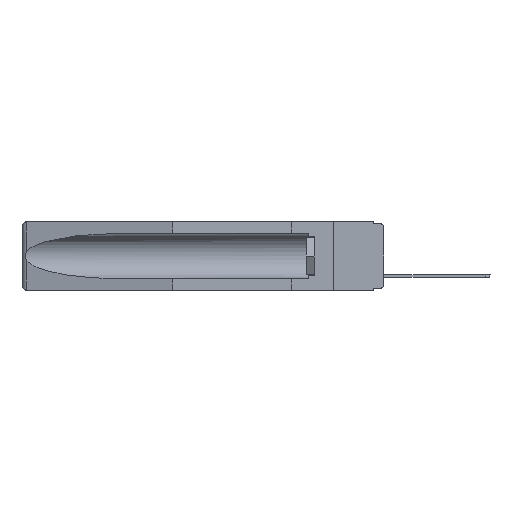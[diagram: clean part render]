
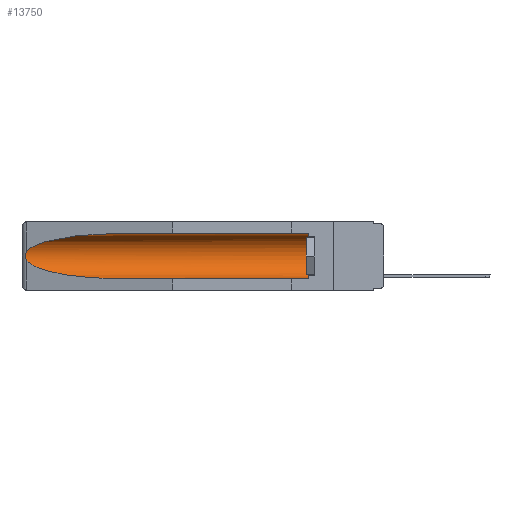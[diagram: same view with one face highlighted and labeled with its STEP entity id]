
A CAD part, left-side view. The second image highlights one B-rep face of the part: STEP entity #13750.
In plain terms, the highlighted cylindrical face has radius 2.857 mm (diameter 5.715 mm), a partial arc.
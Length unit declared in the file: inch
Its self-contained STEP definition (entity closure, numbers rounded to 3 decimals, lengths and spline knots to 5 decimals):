
#1207 = DIRECTION ( 'NONE',  ( 0., 0., 1. ) ) ;
#1569 = ORIENTED_EDGE ( 'NONE', *, *, #2004, .T. ) ;
#1913 = VERTEX_POINT ( 'NONE', #12343 ) ;
#1918 = CARTESIAN_POINT ( 'NONE',  ( 0.155, 1.07973, -0.059 ) ) ;
#1932 = EDGE_CURVE ( 'NONE', #7991, #20715, #3183, .T. ) ;
#2004 = EDGE_CURVE ( 'NONE', #13386, #7965, #2356, .T. ) ;
#2179 = CARTESIAN_POINT ( 'NONE',  ( 0.2673, 1.53269, -0.17917 ) ) ;
#2356 =( BOUNDED_CURVE ( )  B_SPLINE_CURVE ( 3, ( #19872, #16302, #10547, #3403 ),
 .UNSPECIFIED., .F., .F. ) 
 B_SPLINE_CURVE_WITH_KNOTS ( ( 4, 4 ),
 ( 0.1948, 1.5708 ),
 .UNSPECIFIED. ) 
 CURVE ( )  GEOMETRIC_REPRESENTATION_ITEM ( )  RATIONAL_B_SPLINE_CURVE ( ( 1., 0.848, 0.848, 1. ) ) 
 REPRESENTATION_ITEM ( '' )  );
#2680 = VECTOR ( 'NONE', #16336, 39.37008 ) ;
#2897 = DIRECTION ( 'NONE',  ( 0., 0., 1. ) ) ;
#3183 = LINE ( 'NONE', #8618, #13133 ) ;
#3218 = LINE ( 'NONE', #8899, #2680 ) ;
#3403 = CARTESIAN_POINT ( 'NONE',  ( 0.155, 1.07973, -0.284 ) ) ;
#3861 = CARTESIAN_POINT ( 'NONE',  ( 0.2673, 1.5327, -0.16383 ) ) ;
#4506 = DIRECTION ( 'NONE',  ( 0., 1., 0. ) ) ;
#5332 = AXIS2_PLACEMENT_3D ( 'NONE', #14336, #21502, #1207 ) ;
#5434 = CARTESIAN_POINT ( 'NONE',  ( 0.2675, 1.53308, -0.16763 ) ) ;
#5919 = CARTESIAN_POINT ( 'NONE',  ( 0.26597, 1.5296, -0.19026 ) ) ;
#7965 = VERTEX_POINT ( 'NONE', #21753 ) ;
#7991 = VERTEX_POINT ( 'NONE', #19825 ) ;
#8219 = B_SPLINE_CURVE_WITH_KNOTS ( 'NONE', 3,
 ( #22138, #22256, #20326, #3861, #5434, #18418, #2179, #18542, #5919, #16748 ),
 .UNSPECIFIED., .F., .F.,
 ( 4, 2, 2, 2, 4 ),
 ( 0., 0.00029, 0.00058, 0.00087, 0.00117 ),
 .UNSPECIFIED. ) ;
#8432 = CARTESIAN_POINT ( 'NONE',  ( 0.155, 0.126, -0.1715 ) ) ;
#8453 = CIRCLE ( 'NONE', #15736, 0.1125 ) ;
#8618 = CARTESIAN_POINT ( 'NONE',  ( 0.155, -0.30754, -0.059 ) ) ;
#8899 = CARTESIAN_POINT ( 'NONE',  ( 0.155, -0.30754, -0.284 ) ) ;
#9932 = CARTESIAN_POINT ( 'NONE',  ( 0.155, 1.07973, -0.059 ) ) ;
#10547 = CARTESIAN_POINT ( 'NONE',  ( 0.21114, 1.30732, -0.284 ) ) ;
#10597 = ORIENTED_EDGE ( 'NONE', *, *, #23426, .T. ) ;
#10706 = FACE_OUTER_BOUND ( 'NONE', #15155, .T. ) ;
#10861 = ORIENTED_EDGE ( 'NONE', *, *, #20026, .T. ) ;
#10895 = ORIENTED_EDGE ( 'NONE', *, *, #23756, .T. ) ;
#12168 = CYLINDRICAL_SURFACE ( 'NONE', #5332, 0.1125 ) ;
#12343 = CARTESIAN_POINT ( 'NONE',  ( 0.155, 0.126, -0.284 ) ) ;
#13133 = VECTOR ( 'NONE', #4506, 39.37008 ) ;
#13239 = CARTESIAN_POINT ( 'NONE',  ( 0.26537, 1.52718, -0.14972 ) ) ;
#13386 = VERTEX_POINT ( 'NONE', #16242 ) ;
#13750 = ADVANCED_FACE ( 'NONE', ( #10706 ), #12168, .F. ) ;
#14102 = ORIENTED_EDGE ( 'NONE', *, *, #14503, .F. ) ;
#14336 = CARTESIAN_POINT ( 'NONE',  ( 0.155, -0.30754, -0.1715 ) ) ;
#14503 = EDGE_CURVE ( 'NONE', #1913, #7965, #3218, .T. ) ;
#14847 =( BOUNDED_CURVE ( )  B_SPLINE_CURVE ( 3, ( #9932, #15684, #21200, #23125 ),
 .UNSPECIFIED., .F., .F. ) 
 B_SPLINE_CURVE_WITH_KNOTS ( ( 4, 4 ),
 ( 4.71239, 6.08839 ),
 .UNSPECIFIED. ) 
 CURVE ( )  GEOMETRIC_REPRESENTATION_ITEM ( )  RATIONAL_B_SPLINE_CURVE ( ( 1., 0.848, 0.848, 1. ) ) 
 REPRESENTATION_ITEM ( '' )  );
#15155 = EDGE_LOOP ( 'NONE', ( #10861, #10597, #1569, #14102, #10895, #19170 ) ) ;
#15684 = CARTESIAN_POINT ( 'NONE',  ( 0.21114, 1.30732, -0.059 ) ) ;
#15736 = AXIS2_PLACEMENT_3D ( 'NONE', #8432, #15991, #2897 ) ;
#15991 = DIRECTION ( 'NONE',  ( 0., -1., 0. ) ) ;
#16242 = CARTESIAN_POINT ( 'NONE',  ( 0.26537, 1.52718, -0.19328 ) ) ;
#16302 = CARTESIAN_POINT ( 'NONE',  ( 0.25451, 1.48313, -0.24835 ) ) ;
#16336 = DIRECTION ( 'NONE',  ( 0., 1., 0. ) ) ;
#16748 = CARTESIAN_POINT ( 'NONE',  ( 0.26537, 1.52718, -0.19328 ) ) ;
#18418 = CARTESIAN_POINT ( 'NONE',  ( 0.2675, 1.53308, -0.17534 ) ) ;
#18542 = CARTESIAN_POINT ( 'NONE',  ( 0.26655, 1.53094, -0.18657 ) ) ;
#19170 = ORIENTED_EDGE ( 'NONE', *, *, #1932, .T. ) ;
#19825 = CARTESIAN_POINT ( 'NONE',  ( 0.155, 0.126, -0.059 ) ) ;
#19872 = CARTESIAN_POINT ( 'NONE',  ( 0.26537, 1.52718, -0.19328 ) ) ;
#20026 = EDGE_CURVE ( 'NONE', #20715, #22468, #14847, .T. ) ;
#20326 = CARTESIAN_POINT ( 'NONE',  ( 0.26654, 1.53092, -0.15636 ) ) ;
#20715 = VERTEX_POINT ( 'NONE', #1918 ) ;
#21200 = CARTESIAN_POINT ( 'NONE',  ( 0.25451, 1.48313, -0.09465 ) ) ;
#21502 = DIRECTION ( 'NONE',  ( 0., 1., 0. ) ) ;
#21753 = CARTESIAN_POINT ( 'NONE',  ( 0.155, 1.07973, -0.284 ) ) ;
#22138 = CARTESIAN_POINT ( 'NONE',  ( 0.26537, 1.52718, -0.14972 ) ) ;
#22256 = CARTESIAN_POINT ( 'NONE',  ( 0.26597, 1.52961, -0.15275 ) ) ;
#22468 = VERTEX_POINT ( 'NONE', #13239 ) ;
#23125 = CARTESIAN_POINT ( 'NONE',  ( 0.26537, 1.52718, -0.14972 ) ) ;
#23426 = EDGE_CURVE ( 'NONE', #22468, #13386, #8219, .T. ) ;
#23756 = EDGE_CURVE ( 'NONE', #1913, #7991, #8453, .T. ) ;
